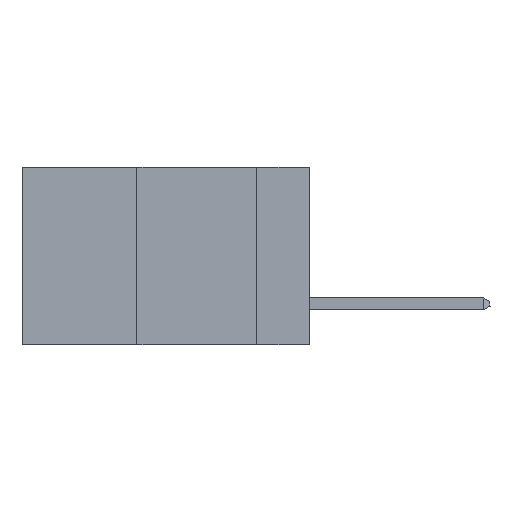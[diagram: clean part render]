
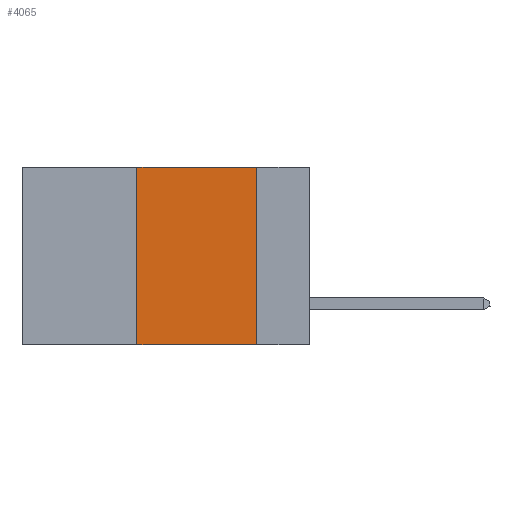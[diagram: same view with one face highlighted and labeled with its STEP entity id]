
A CAD part, left-side view. The second image highlights one B-rep face of the part: STEP entity #4065.
In plain terms, the highlighted planar face has unit normal (-1, 0, 0).
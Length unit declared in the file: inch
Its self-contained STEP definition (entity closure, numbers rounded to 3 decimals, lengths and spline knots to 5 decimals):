
#334 = CARTESIAN_POINT ( 'NONE',  ( 0., 0.6, 0. ) ) ;
#822 = VERTEX_POINT ( 'NONE', #7969 ) ;
#1067 = EDGE_CURVE ( 'NONE', #1309, #10203, #9181, .T. ) ;
#1309 = VERTEX_POINT ( 'NONE', #15346 ) ;
#1803 = ORIENTED_EDGE ( 'NONE', *, *, #2655, .F. ) ;
#1960 = VECTOR ( 'NONE', #4517, 39.37008 ) ;
#2345 = DIRECTION ( 'NONE',  ( 0., 0., -1. ) ) ;
#2655 = EDGE_CURVE ( 'NONE', #10203, #822, #13349, .T. ) ;
#2695 = CARTESIAN_POINT ( 'NONE',  ( 0., 0.6, -0.37 ) ) ;
#2832 = EDGE_CURVE ( 'NONE', #822, #10401, #16700, .T. ) ;
#3540 = DIRECTION ( 'NONE',  ( 1., 0., 0. ) ) ;
#4008 = FACE_OUTER_BOUND ( 'NONE', #10068, .T. ) ;
#4065 = ADVANCED_FACE ( 'NONE', ( #4008 ), #7801, .F. ) ;
#4517 = DIRECTION ( 'NONE',  ( 0., 0., 1. ) ) ;
#5469 = AXIS2_PLACEMENT_3D ( 'NONE', #7679, #3540, #2345 ) ;
#5539 = DIRECTION ( 'NONE',  ( 0., -1., 0. ) ) ;
#7461 = DIRECTION ( 'NONE',  ( 0., 0., -1. ) ) ;
#7679 = CARTESIAN_POINT ( 'NONE',  ( 0., 0.6, 0. ) ) ;
#7685 = CARTESIAN_POINT ( 'NONE',  ( 0., 0.11, 0. ) ) ;
#7801 = PLANE ( 'NONE',  #5469 ) ;
#7969 = CARTESIAN_POINT ( 'NONE',  ( 0., 0.11, 0. ) ) ;
#8305 = EDGE_CURVE ( 'NONE', #1309, #10401, #13248, .T. ) ;
#8351 = ORIENTED_EDGE ( 'NONE', *, *, #1067, .F. ) ;
#9171 = CARTESIAN_POINT ( 'NONE',  ( 0., 0.11, -0.37 ) ) ;
#9181 = LINE ( 'NONE', #12471, #1960 ) ;
#9415 = ORIENTED_EDGE ( 'NONE', *, *, #8305, .T. ) ;
#10068 = EDGE_LOOP ( 'NONE', ( #11593, #1803, #8351, #9415 ) ) ;
#10203 = VERTEX_POINT ( 'NONE', #13023 ) ;
#10294 = VECTOR ( 'NONE', #5539, 39.37008 ) ;
#10401 = VERTEX_POINT ( 'NONE', #9171 ) ;
#11593 = ORIENTED_EDGE ( 'NONE', *, *, #2832, .F. ) ;
#12471 = CARTESIAN_POINT ( 'NONE',  ( 0., 0.36, 0. ) ) ;
#12775 = DIRECTION ( 'NONE',  ( 0., -1., 0. ) ) ;
#13023 = CARTESIAN_POINT ( 'NONE',  ( 0., 0.36, 0. ) ) ;
#13248 = LINE ( 'NONE', #2695, #10294 ) ;
#13349 = LINE ( 'NONE', #334, #15038 ) ;
#15038 = VECTOR ( 'NONE', #12775, 39.37008 ) ;
#15241 = VECTOR ( 'NONE', #7461, 39.37008 ) ;
#15346 = CARTESIAN_POINT ( 'NONE',  ( 0., 0.36, -0.37 ) ) ;
#16700 = LINE ( 'NONE', #7685, #15241 ) ;
